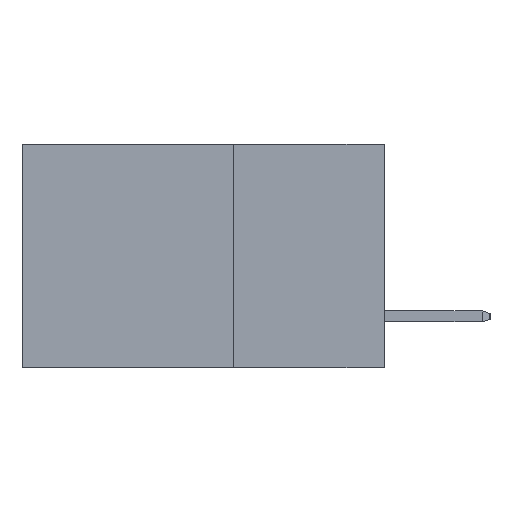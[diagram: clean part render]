
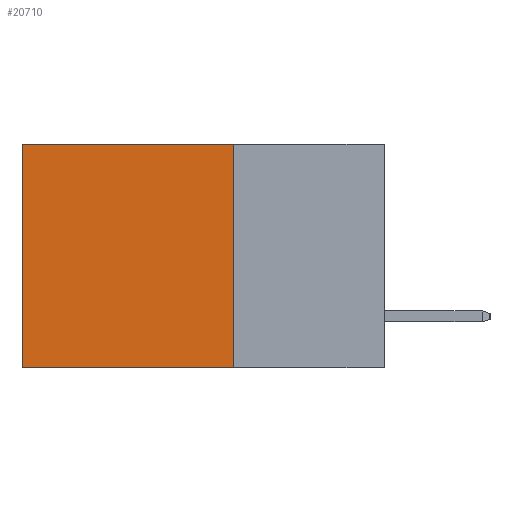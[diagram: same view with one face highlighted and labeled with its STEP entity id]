
A CAD part, left-side view. The second image highlights one B-rep face of the part: STEP entity #20710.
In plain terms, the highlighted planar face has unit normal (-1, 0, 0).
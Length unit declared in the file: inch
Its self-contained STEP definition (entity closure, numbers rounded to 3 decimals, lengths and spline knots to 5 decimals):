
#737 = DIRECTION ( 'NONE',  ( 0., 0., -1. ) ) ;
#1599 = DIRECTION ( 'NONE',  ( 0., 1., 0. ) ) ;
#2114 = DIRECTION ( 'NONE',  ( 0., 0., -1. ) ) ;
#2207 = CARTESIAN_POINT ( 'NONE',  ( 0.298, 0.25, 0. ) ) ;
#2225 = VECTOR ( 'NONE', #1599, 39.37008 ) ;
#3860 = EDGE_LOOP ( 'NONE', ( #24403, #18110, #13382, #17336 ) ) ;
#3918 = VERTEX_POINT ( 'NONE', #2207 ) ;
#4184 = CARTESIAN_POINT ( 'NONE',  ( 0.298, 0.6, -0.37 ) ) ;
#5088 = CARTESIAN_POINT ( 'NONE',  ( 0.298, 0.6, 0. ) ) ;
#6168 = VECTOR ( 'NONE', #2114, 39.37008 ) ;
#6214 = EDGE_CURVE ( 'NONE', #15052, #16792, #7108, .T. ) ;
#7072 = EDGE_CURVE ( 'NONE', #3918, #15981, #11364, .T. ) ;
#7108 = LINE ( 'NONE', #5088, #16798 ) ;
#7190 = DIRECTION ( 'NONE',  ( 0., 0., -1. ) ) ;
#7860 = DIRECTION ( 'NONE',  ( 0., 1., 0. ) ) ;
#9597 = VECTOR ( 'NONE', #7860, 39.37008 ) ;
#10889 = FACE_OUTER_BOUND ( 'NONE', #3860, .T. ) ;
#11174 = EDGE_CURVE ( 'NONE', #3918, #15052, #14771, .T. ) ;
#11364 = LINE ( 'NONE', #19594, #6168 ) ;
#13344 = CARTESIAN_POINT ( 'NONE',  ( 0.298, 0.25, -0.37 ) ) ;
#13382 = ORIENTED_EDGE ( 'NONE', *, *, #7072, .F. ) ;
#13445 = EDGE_CURVE ( 'NONE', #15981, #16792, #19612, .T. ) ;
#14771 = LINE ( 'NONE', #19457, #9597 ) ;
#15052 = VERTEX_POINT ( 'NONE', #20441 ) ;
#15981 = VERTEX_POINT ( 'NONE', #13344 ) ;
#16792 = VERTEX_POINT ( 'NONE', #4184 ) ;
#16798 = VECTOR ( 'NONE', #737, 39.37008 ) ;
#17176 = AXIS2_PLACEMENT_3D ( 'NONE', #22574, #18833, #7190 ) ;
#17336 = ORIENTED_EDGE ( 'NONE', *, *, #11174, .T. ) ;
#18110 = ORIENTED_EDGE ( 'NONE', *, *, #13445, .F. ) ;
#18753 = PLANE ( 'NONE',  #17176 ) ;
#18833 = DIRECTION ( 'NONE',  ( 1., 0., 0. ) ) ;
#19457 = CARTESIAN_POINT ( 'NONE',  ( 0.298, 0.25, 0. ) ) ;
#19594 = CARTESIAN_POINT ( 'NONE',  ( 0.298, 0.25, 0. ) ) ;
#19612 = LINE ( 'NONE', #22843, #2225 ) ;
#20441 = CARTESIAN_POINT ( 'NONE',  ( 0.298, 0.6, 0. ) ) ;
#20710 = ADVANCED_FACE ( 'NONE', ( #10889 ), #18753, .F. ) ;
#22574 = CARTESIAN_POINT ( 'NONE',  ( 0.298, 0.25, 0. ) ) ;
#22843 = CARTESIAN_POINT ( 'NONE',  ( 0.298, 0.25, -0.37 ) ) ;
#24403 = ORIENTED_EDGE ( 'NONE', *, *, #6214, .T. ) ;
